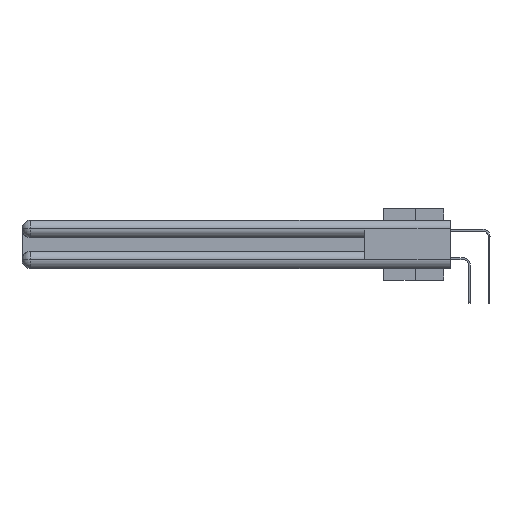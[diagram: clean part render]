
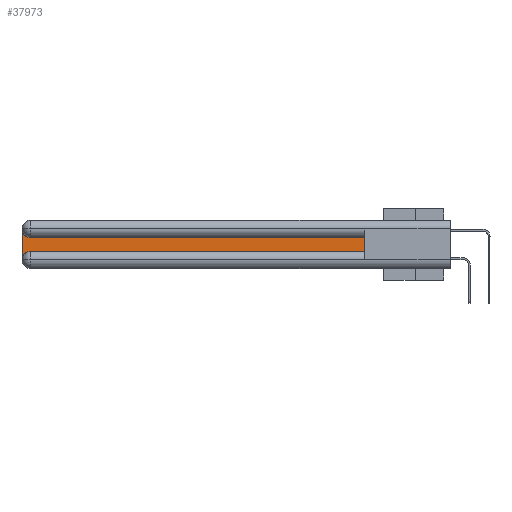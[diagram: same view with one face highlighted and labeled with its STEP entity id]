
A CAD part, left-side view. The second image highlights one B-rep face of the part: STEP entity #37973.
In plain terms, the highlighted planar face has unit normal (-1, 0, 0).
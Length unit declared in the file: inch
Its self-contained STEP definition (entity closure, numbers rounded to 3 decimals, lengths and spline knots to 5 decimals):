
#418 = CARTESIAN_POINT ( 'NONE',  ( 0.075, 3., -0.0625 ) ) ;
#1533 = LINE ( 'NONE', #37434, #40125 ) ;
#2229 = CARTESIAN_POINT ( 'NONE',  ( 0.075, 0.6, -0.1225 ) ) ;
#4616 = DIRECTION ( 'NONE',  ( 0., 0., -1. ) ) ;
#4742 = CARTESIAN_POINT ( 'NONE',  ( 0.075, 0.6, -0.2175 ) ) ;
#4958 = DIRECTION ( 'NONE',  ( 0., 0., 1. ) ) ;
#5054 = CARTESIAN_POINT ( 'NONE',  ( 0.075, 2.94, -0.0625 ) ) ;
#5192 = CARTESIAN_POINT ( 'NONE',  ( 0.075, 0.6, -0.1225 ) ) ;
#5479 = ORIENTED_EDGE ( 'NONE', *, *, #9630, .T. ) ;
#5652 = CARTESIAN_POINT ( 'NONE',  ( 0.075, 2.94, -0.2175 ) ) ;
#5977 = VERTEX_POINT ( 'NONE', #13307 ) ;
#6479 = DIRECTION ( 'NONE',  ( 0., 0., -1. ) ) ;
#6979 = EDGE_LOOP ( 'NONE', ( #9525, #37564, #33525, #11293, #17345, #5479 ) ) ;
#7829 = DIRECTION ( 'NONE',  ( 1., 0., 0. ) ) ;
#8038 = FACE_OUTER_BOUND ( 'NONE', #6979, .T. ) ;
#9162 = EDGE_CURVE ( 'NONE', #34022, #5977, #37905, .T. ) ;
#9525 = ORIENTED_EDGE ( 'NONE', *, *, #9162, .T. ) ;
#9630 = EDGE_CURVE ( 'NONE', #27869, #34022, #34213, .T. ) ;
#11293 = ORIENTED_EDGE ( 'NONE', *, *, #25744, .T. ) ;
#12086 = EDGE_CURVE ( 'NONE', #5977, #27760, #22768, .T. ) ;
#12245 = CIRCLE ( 'NONE', #27258, 0.06 ) ;
#12921 = DIRECTION ( 'NONE',  ( 1., 0., 0. ) ) ;
#13307 = CARTESIAN_POINT ( 'NONE',  ( 0.075, 2.94, -0.1225 ) ) ;
#14474 = VECTOR ( 'NONE', #34685, 39.37008 ) ;
#15921 = CARTESIAN_POINT ( 'NONE',  ( 0.075, 2.94, -0.2775 ) ) ;
#17345 = ORIENTED_EDGE ( 'NONE', *, *, #23991, .T. ) ;
#22581 = DIRECTION ( 'NONE',  ( 0., -1., 0. ) ) ;
#22768 = CIRCLE ( 'NONE', #34374, 0.06 ) ;
#23376 = VECTOR ( 'NONE', #4958, 39.37008 ) ;
#23406 = LINE ( 'NONE', #29627, #38134 ) ;
#23862 = DIRECTION ( 'NONE',  ( 0., 0., -1. ) ) ;
#23991 = EDGE_CURVE ( 'NONE', #25690, #27869, #23406, .T. ) ;
#24060 = AXIS2_PLACEMENT_3D ( 'NONE', #33883, #7829, #4616 ) ;
#24682 = EDGE_CURVE ( 'NONE', #27760, #30300, #1533, .T. ) ;
#25690 = VERTEX_POINT ( 'NONE', #5652 ) ;
#25744 = EDGE_CURVE ( 'NONE', #30300, #25690, #12245, .T. ) ;
#27258 = AXIS2_PLACEMENT_3D ( 'NONE', #15921, #12921, #6479 ) ;
#27760 = VERTEX_POINT ( 'NONE', #418 ) ;
#27869 = VERTEX_POINT ( 'NONE', #31013 ) ;
#29627 = CARTESIAN_POINT ( 'NONE',  ( 0.075, 0.6, -0.2175 ) ) ;
#30300 = VERTEX_POINT ( 'NONE', #32547 ) ;
#30704 = DIRECTION ( 'NONE',  ( 1., 0., 0. ) ) ;
#31013 = CARTESIAN_POINT ( 'NONE',  ( 0.075, 0.6, -0.2175 ) ) ;
#32547 = CARTESIAN_POINT ( 'NONE',  ( 0.075, 3., -0.2775 ) ) ;
#33525 = ORIENTED_EDGE ( 'NONE', *, *, #24682, .T. ) ;
#33883 = CARTESIAN_POINT ( 'NONE',  ( 0.075, 3., -0.1225 ) ) ;
#34022 = VERTEX_POINT ( 'NONE', #5192 ) ;
#34213 = LINE ( 'NONE', #4742, #23376 ) ;
#34374 = AXIS2_PLACEMENT_3D ( 'NONE', #5054, #30704, #23862 ) ;
#34685 = DIRECTION ( 'NONE',  ( 0., 1., 0. ) ) ;
#35062 = DIRECTION ( 'NONE',  ( 0., 0., -1. ) ) ;
#37095 = PLANE ( 'NONE',  #24060 ) ;
#37434 = CARTESIAN_POINT ( 'NONE',  ( 0.075, 3., -0.2175 ) ) ;
#37564 = ORIENTED_EDGE ( 'NONE', *, *, #12086, .T. ) ;
#37905 = LINE ( 'NONE', #2229, #14474 ) ;
#37973 = ADVANCED_FACE ( 'NONE', ( #8038 ), #37095, .F. ) ;
#38134 = VECTOR ( 'NONE', #22581, 39.37008 ) ;
#40125 = VECTOR ( 'NONE', #35062, 39.37008 ) ;
